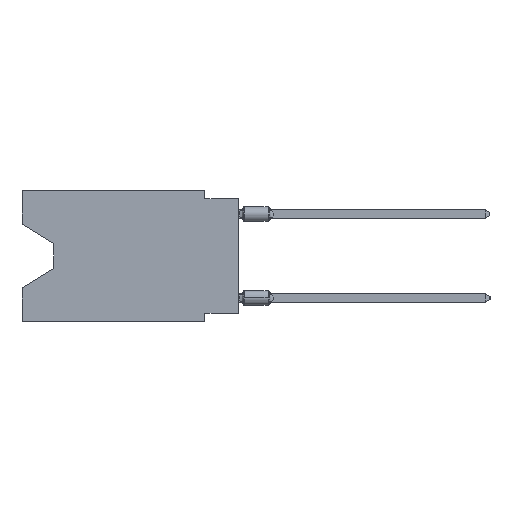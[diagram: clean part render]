
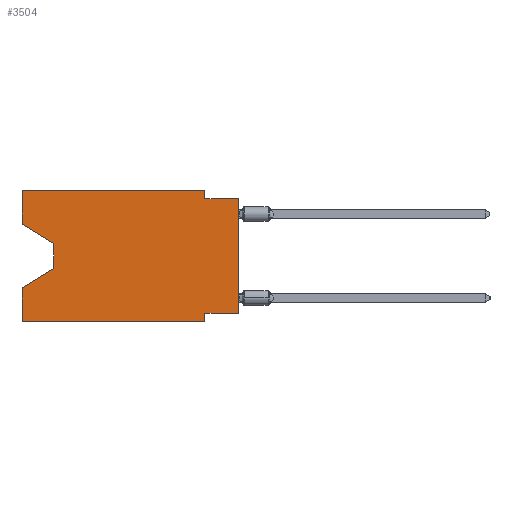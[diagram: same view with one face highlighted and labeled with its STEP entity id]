
A CAD part, left-side view. The second image highlights one B-rep face of the part: STEP entity #3504.
In plain terms, the highlighted planar face has unit normal (-1, 0, 0).
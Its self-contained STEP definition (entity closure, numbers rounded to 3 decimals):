
#316 = DIRECTION ( 'NONE',  ( 0., 0., -1. ) ) ;
#721 = VERTEX_POINT ( 'NONE', #32987 ) ;
#780 = LINE ( 'NONE', #49612, #4035 ) ;
#938 = CARTESIAN_POINT ( 'NONE',  ( 0., 16.383, -9.906 ) ) ;
#3157 = DIRECTION ( 'NONE',  ( 0., 0., 1. ) ) ;
#3504 = ADVANCED_FACE ( 'NONE', ( #22520 ), #31304, .F. ) ;
#4035 = VECTOR ( 'NONE', #45225, 1000. ) ;
#4696 = LINE ( 'NONE', #40668, #47784 ) ;
#5240 = LINE ( 'NONE', #31295, #44850 ) ;
#5621 = ORIENTED_EDGE ( 'NONE', *, *, #52335, .T. ) ;
#6870 = CARTESIAN_POINT ( 'NONE',  ( 0., 2.54, -9.906 ) ) ;
#7049 = VECTOR ( 'NONE', #36502, 1000. ) ;
#7442 = ORIENTED_EDGE ( 'NONE', *, *, #51997, .F. ) ;
#7576 = VERTEX_POINT ( 'NONE', #56256 ) ;
#8396 = LINE ( 'NONE', #47885, #15508 ) ;
#8794 = VECTOR ( 'NONE', #53790, 1000. ) ;
#9046 = LINE ( 'NONE', #35940, #8794 ) ;
#9233 = EDGE_CURVE ( 'NONE', #27780, #44306, #44706, .T. ) ;
#11007 = LINE ( 'NONE', #46658, #42677 ) ;
#11118 = EDGE_CURVE ( 'NONE', #46378, #34311, #780, .T. ) ;
#13142 = VECTOR ( 'NONE', #37179, 1000. ) ;
#13464 = DIRECTION ( 'NONE',  ( 0., -1., 0. ) ) ;
#14976 = ORIENTED_EDGE ( 'NONE', *, *, #15960, .F. ) ;
#15158 = EDGE_CURVE ( 'NONE', #45402, #21197, #5240, .T. ) ;
#15508 = VECTOR ( 'NONE', #3157, 1000. ) ;
#15960 = EDGE_CURVE ( 'NONE', #45402, #721, #42396, .T. ) ;
#16171 = EDGE_CURVE ( 'NONE', #34311, #21535, #4696, .T. ) ;
#17094 = CARTESIAN_POINT ( 'NONE',  ( 0., 16.383, -2.546 ) ) ;
#17295 = CARTESIAN_POINT ( 'NONE',  ( 0., 16.383, 0. ) ) ;
#17309 = ORIENTED_EDGE ( 'NONE', *, *, #53858, .F. ) ;
#17910 = EDGE_CURVE ( 'NONE', #21535, #721, #9046, .T. ) ;
#18425 = DIRECTION ( 'NONE',  ( 0., -1., 0. ) ) ;
#18773 = VECTOR ( 'NONE', #13464, 1000. ) ;
#19624 = CARTESIAN_POINT ( 'NONE',  ( 0., 2.54, -0.635 ) ) ;
#20763 = ORIENTED_EDGE ( 'NONE', *, *, #31171, .F. ) ;
#21197 = VERTEX_POINT ( 'NONE', #6870 ) ;
#21349 = DIRECTION ( 'NONE',  ( 0., 0., 1. ) ) ;
#21535 = VERTEX_POINT ( 'NONE', #49503 ) ;
#21647 = VECTOR ( 'NONE', #21349, 1000. ) ;
#21968 = DIRECTION ( 'NONE',  ( 1., 0., 0. ) ) ;
#22389 = ORIENTED_EDGE ( 'NONE', *, *, #16171, .T. ) ;
#22520 = FACE_OUTER_BOUND ( 'NONE', #33761, .T. ) ;
#24712 = ORIENTED_EDGE ( 'NONE', *, *, #15158, .T. ) ;
#27780 = VERTEX_POINT ( 'NONE', #19624 ) ;
#28279 = DIRECTION ( 'NONE',  ( 0., 0., 1. ) ) ;
#30308 = LINE ( 'NONE', #34955, #42158 ) ;
#30896 = VERTEX_POINT ( 'NONE', #51654 ) ;
#31171 = EDGE_CURVE ( 'NONE', #54956, #7576, #41567, .T. ) ;
#31295 = CARTESIAN_POINT ( 'NONE',  ( 0., 16.383, -9.906 ) ) ;
#31304 = PLANE ( 'NONE',  #42645 ) ;
#32987 = CARTESIAN_POINT ( 'NONE',  ( 0., 16.383, -7.36 ) ) ;
#33761 = EDGE_LOOP ( 'NONE', ( #55270, #22389, #49610, #14976, #24712, #49520, #7442, #5621, #35051, #50421, #20763, #17309 ) ) ;
#34311 = VERTEX_POINT ( 'NONE', #38452 ) ;
#34955 = CARTESIAN_POINT ( 'NONE',  ( 0., 2.54, 0. ) ) ;
#35051 = ORIENTED_EDGE ( 'NONE', *, *, #9233, .F. ) ;
#35940 = CARTESIAN_POINT ( 'NONE',  ( 0., 13.97, -5.893 ) ) ;
#36502 = DIRECTION ( 'NONE',  ( 0., 1., 0. ) ) ;
#37179 = DIRECTION ( 'NONE',  ( 0., -1., 0. ) ) ;
#37599 = EDGE_CURVE ( 'NONE', #7576, #27780, #30308, .T. ) ;
#38010 = VECTOR ( 'NONE', #45744, 1000. ) ;
#38291 = CARTESIAN_POINT ( 'NONE',  ( 0., 16.383, 0. ) ) ;
#38452 = CARTESIAN_POINT ( 'NONE',  ( 0., 13.97, -4.013 ) ) ;
#39169 = CARTESIAN_POINT ( 'NONE',  ( 0., 0., -0.635 ) ) ;
#40668 = CARTESIAN_POINT ( 'NONE',  ( 0., 13.97, -4.013 ) ) ;
#41077 = CARTESIAN_POINT ( 'NONE',  ( 0., 2.54, -9.906 ) ) ;
#41567 = LINE ( 'NONE', #55024, #13142 ) ;
#41946 = LINE ( 'NONE', #41077, #38010 ) ;
#42158 = VECTOR ( 'NONE', #45147, 1000. ) ;
#42396 = LINE ( 'NONE', #38291, #21647 ) ;
#42645 = AXIS2_PLACEMENT_3D ( 'NONE', #17295, #21968, #52947 ) ;
#42677 = VECTOR ( 'NONE', #28279, 1000. ) ;
#44040 = CARTESIAN_POINT ( 'NONE',  ( 0., 2.54, -9.271 ) ) ;
#44306 = VERTEX_POINT ( 'NONE', #50339 ) ;
#44428 = CARTESIAN_POINT ( 'NONE',  ( 0., 0., -9.271 ) ) ;
#44700 = LINE ( 'NONE', #44428, #7049 ) ;
#44706 = LINE ( 'NONE', #39169, #18773 ) ;
#44850 = VECTOR ( 'NONE', #18425, 1000. ) ;
#45147 = DIRECTION ( 'NONE',  ( 0., 0., -1. ) ) ;
#45225 = DIRECTION ( 'NONE',  ( 0., -0.855, -0.519 ) ) ;
#45402 = VERTEX_POINT ( 'NONE', #938 ) ;
#45744 = DIRECTION ( 'NONE',  ( 0., 0., -1. ) ) ;
#46378 = VERTEX_POINT ( 'NONE', #17094 ) ;
#46658 = CARTESIAN_POINT ( 'NONE',  ( 0., 16.383, 0. ) ) ;
#47784 = VECTOR ( 'NONE', #316, 1000. ) ;
#47885 = CARTESIAN_POINT ( 'NONE',  ( 0., 0., 0. ) ) ;
#49503 = CARTESIAN_POINT ( 'NONE',  ( 0., 13.97, -5.893 ) ) ;
#49520 = ORIENTED_EDGE ( 'NONE', *, *, #55793, .F. ) ;
#49610 = ORIENTED_EDGE ( 'NONE', *, *, #17910, .T. ) ;
#49612 = CARTESIAN_POINT ( 'NONE',  ( 0., 16.383, -2.546 ) ) ;
#50339 = CARTESIAN_POINT ( 'NONE',  ( 0., 0., -0.635 ) ) ;
#50421 = ORIENTED_EDGE ( 'NONE', *, *, #37599, .F. ) ;
#51654 = CARTESIAN_POINT ( 'NONE',  ( 0., 0., -9.271 ) ) ;
#51997 = EDGE_CURVE ( 'NONE', #30896, #55696, #44700, .T. ) ;
#52335 = EDGE_CURVE ( 'NONE', #30896, #44306, #8396, .T. ) ;
#52947 = DIRECTION ( 'NONE',  ( 0., 0., -1. ) ) ;
#53790 = DIRECTION ( 'NONE',  ( 0., 0.855, -0.519 ) ) ;
#53858 = EDGE_CURVE ( 'NONE', #46378, #54956, #11007, .T. ) ;
#54020 = CARTESIAN_POINT ( 'NONE',  ( 0., 16.383, 0. ) ) ;
#54956 = VERTEX_POINT ( 'NONE', #54020 ) ;
#55024 = CARTESIAN_POINT ( 'NONE',  ( 0., 16.383, 0. ) ) ;
#55270 = ORIENTED_EDGE ( 'NONE', *, *, #11118, .T. ) ;
#55696 = VERTEX_POINT ( 'NONE', #44040 ) ;
#55793 = EDGE_CURVE ( 'NONE', #55696, #21197, #41946, .T. ) ;
#56256 = CARTESIAN_POINT ( 'NONE',  ( 0., 2.54, 0. ) ) ;
